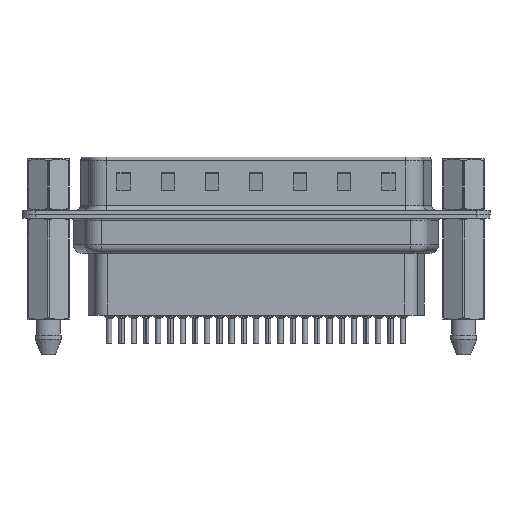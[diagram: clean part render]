
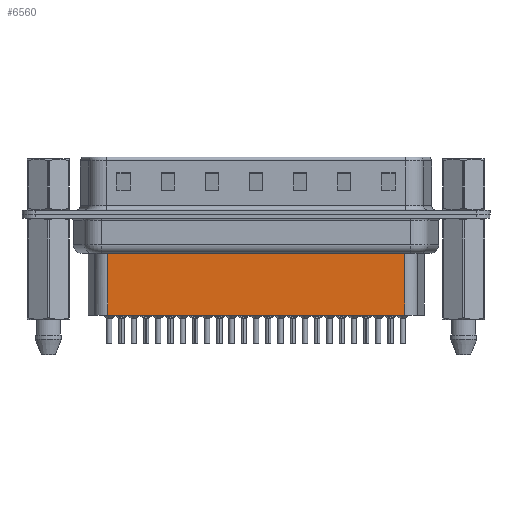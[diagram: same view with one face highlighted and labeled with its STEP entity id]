
A CAD part, front view. The second image highlights one B-rep face of the part: STEP entity #6560.
In plain terms, the highlighted planar face has unit normal (0, -1, 0).
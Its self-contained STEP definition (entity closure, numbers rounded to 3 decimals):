
#925 = LINE ( 'NONE', #24322, #13670 ) ;
#1517 = VERTEX_POINT ( 'NONE', #18881 ) ;
#1673 = CARTESIAN_POINT ( 'NONE',  ( 6.706, -3.5, -3.1 ) ) ;
#1816 = AXIS2_PLACEMENT_3D ( 'NONE', #24541, #8677, #26387 ) ;
#2232 = CARTESIAN_POINT ( 'NONE',  ( 6.706, -3.5, -4.097 ) ) ;
#4319 = EDGE_CURVE ( 'NONE', #15574, #1517, #925, .T. ) ;
#6258 = ORIENTED_EDGE ( 'NONE', *, *, #4319, .F. ) ;
#6560 = ADVANCED_FACE ( 'NONE', ( #22160 ), #8787, .T. ) ;
#7651 = ORIENTED_EDGE ( 'NONE', *, *, #27135, .F. ) ;
#8677 = DIRECTION ( 'NONE',  ( 0., -1., 0. ) ) ;
#8787 = PLANE ( 'NONE',  #1816 ) ;
#9189 = CARTESIAN_POINT ( 'NONE',  ( 40.344, -3.5, -4.097 ) ) ;
#9384 = LINE ( 'NONE', #1673, #16140 ) ;
#9855 = VERTEX_POINT ( 'NONE', #9189 ) ;
#10672 = EDGE_CURVE ( 'NONE', #9855, #19963, #17768, .T. ) ;
#12134 = VECTOR ( 'NONE', #20297, 1000. ) ;
#12533 = CARTESIAN_POINT ( 'NONE',  ( 40.344, -3.5, -11.45 ) ) ;
#12618 = CARTESIAN_POINT ( 'NONE',  ( 6.459, -3.5, -4.097 ) ) ;
#13670 = VECTOR ( 'NONE', #24288, 1000. ) ;
#15574 = VERTEX_POINT ( 'NONE', #12533 ) ;
#16140 = VECTOR ( 'NONE', #24180, 1000. ) ;
#17009 = VECTOR ( 'NONE', #20123, 1000. ) ;
#17768 = LINE ( 'NONE', #12618, #17009 ) ;
#17849 = CARTESIAN_POINT ( 'NONE',  ( 40.344, -3.5, -3.1 ) ) ;
#18881 = CARTESIAN_POINT ( 'NONE',  ( 6.706, -3.5, -11.45 ) ) ;
#19963 = VERTEX_POINT ( 'NONE', #2232 ) ;
#20123 = DIRECTION ( 'NONE',  ( -1., 0., 0. ) ) ;
#20297 = DIRECTION ( 'NONE',  ( 0., 0., -1. ) ) ;
#20419 = ORIENTED_EDGE ( 'NONE', *, *, #26392, .T. ) ;
#22160 = FACE_OUTER_BOUND ( 'NONE', #24320, .T. ) ;
#24180 = DIRECTION ( 'NONE',  ( 0., 0., -1. ) ) ;
#24288 = DIRECTION ( 'NONE',  ( -1., 0., 0. ) ) ;
#24320 = EDGE_LOOP ( 'NONE', ( #7651, #25121, #20419, #6258 ) ) ;
#24322 = CARTESIAN_POINT ( 'NONE',  ( 6.706, -3.5, -11.45 ) ) ;
#24541 = CARTESIAN_POINT ( 'NONE',  ( 6.706, -3.5, -3.1 ) ) ;
#25121 = ORIENTED_EDGE ( 'NONE', *, *, #10672, .T. ) ;
#25340 = LINE ( 'NONE', #17849, #12134 ) ;
#26387 = DIRECTION ( 'NONE',  ( 1., 0., 0. ) ) ;
#26392 = EDGE_CURVE ( 'NONE', #19963, #1517, #9384, .T. ) ;
#27135 = EDGE_CURVE ( 'NONE', #9855, #15574, #25340, .T. ) ;
